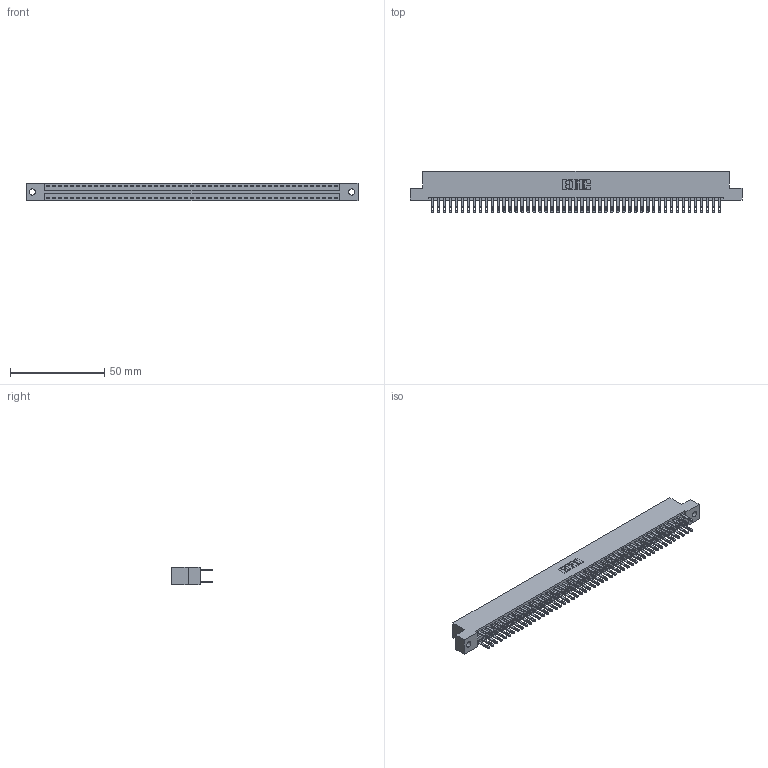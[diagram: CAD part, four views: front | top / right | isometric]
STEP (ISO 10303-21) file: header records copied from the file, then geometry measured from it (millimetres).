
FILE_DESCRIPTION (( 'STEP AP203' ), '1' );
FILE_NAME ('346-098-500-202.STEP', '2022-05-26T17:29:13', ( '' ), ( '' ), 'SwSTEP 2.0', 'SolidWorks 2020', '' );
FILE_SCHEMA (( 'CONFIG_CONTROL_DESIGN' ));
Length unit declared in the file: inch
Products named in the file (3): 346 Part_Flush Mounting Lugs - 0.128 Dia; 346-098-500-202; 345-292-001_345-293-100
Assembly tree (99 placements, depth 2):
  346-098-500-202
    346 Part_Flush Mounting Lugs - 0.128 Dia
    345-292-001_345-293-100  x98
Bounding box: 176.15 x 21.84 x 9.4 mm (x, y, z)
Volume: 17493.9 mm3; surface area: 24913 mm2
Topology: 99 solids, 99 shells, 4826 faces, 14735 edges, 9822 vertices
Faces by surface type: plane 2918, cylinder 1908
Entity records: 30969 total; most frequent: CARTESIAN_POINT 5092, ORIENTED_EDGE 5026, DIRECTION 4541, EDGE_CURVE 2513, LINE 2181, VECTOR 2181, VERTEX_POINT 1674, AXIS2_PLACEMENT_3D 1180
